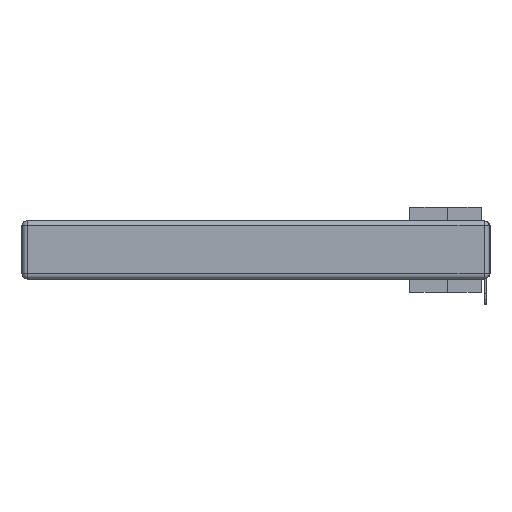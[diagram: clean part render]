
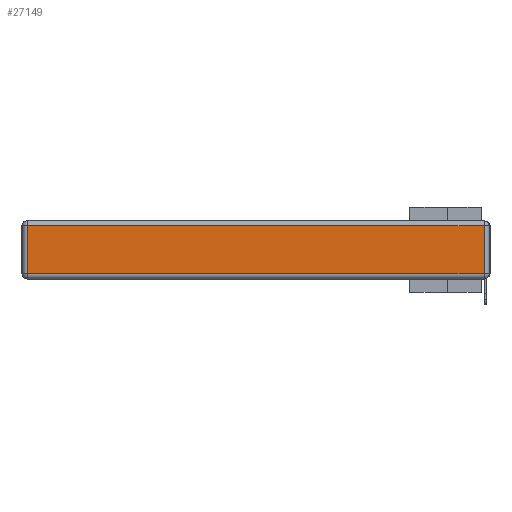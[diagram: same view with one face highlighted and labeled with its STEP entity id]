
A CAD part, left-side view. The second image highlights one B-rep face of the part: STEP entity #27149.
In plain terms, the highlighted planar face has unit normal (-1, 0, 0).
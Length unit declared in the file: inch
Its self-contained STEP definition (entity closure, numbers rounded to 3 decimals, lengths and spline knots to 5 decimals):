
#456 = CARTESIAN_POINT ( 'NONE',  ( 0., 0., -0.313 ) ) ;
#1073 = CARTESIAN_POINT ( 'NONE',  ( 0., 2.72, -0.343 ) ) ;
#1402 = ORIENTED_EDGE ( 'NONE', *, *, #16604, .T. ) ;
#3430 = EDGE_LOOP ( 'NONE', ( #16797, #22699, #1402, #30811 ) ) ;
#3809 = DIRECTION ( 'NONE',  ( 0., 1., 0. ) ) ;
#4510 = VECTOR ( 'NONE', #29214, 39.37008 ) ;
#4762 = CARTESIAN_POINT ( 'NONE',  ( 0., 2.72, -0.03 ) ) ;
#6203 = DIRECTION ( 'NONE',  ( 0., 0., -1. ) ) ;
#6342 = DIRECTION ( 'NONE',  ( 0., 0., 1. ) ) ;
#6616 = VERTEX_POINT ( 'NONE', #13841 ) ;
#13573 = CARTESIAN_POINT ( 'NONE',  ( 0., 0.03, -0.313 ) ) ;
#13841 = CARTESIAN_POINT ( 'NONE',  ( 0., 2.72, -0.313 ) ) ;
#15039 = EDGE_CURVE ( 'NONE', #6616, #26564, #16001, .T. ) ;
#16001 = LINE ( 'NONE', #456, #4510 ) ;
#16604 = EDGE_CURVE ( 'NONE', #32747, #22428, #21941, .T. ) ;
#16797 = ORIENTED_EDGE ( 'NONE', *, *, #15039, .T. ) ;
#17146 = LINE ( 'NONE', #22126, #30282 ) ;
#19828 = PLANE ( 'NONE',  #27016 ) ;
#21829 = EDGE_CURVE ( 'NONE', #22428, #6616, #24355, .T. ) ;
#21941 = LINE ( 'NONE', #32589, #24832 ) ;
#22126 = CARTESIAN_POINT ( 'NONE',  ( 0., 0.03, -0.343 ) ) ;
#22428 = VERTEX_POINT ( 'NONE', #4762 ) ;
#22699 = ORIENTED_EDGE ( 'NONE', *, *, #28020, .T. ) ;
#24355 = LINE ( 'NONE', #1073, #28858 ) ;
#24832 = VECTOR ( 'NONE', #3809, 39.37008 ) ;
#26564 = VERTEX_POINT ( 'NONE', #13573 ) ;
#27016 = AXIS2_PLACEMENT_3D ( 'NONE', #27732, #32885, #6342 ) ;
#27043 = FACE_OUTER_BOUND ( 'NONE', #3430, .T. ) ;
#27149 = ADVANCED_FACE ( 'NONE', ( #27043 ), #19828, .T. ) ;
#27732 = CARTESIAN_POINT ( 'NONE',  ( 0., 0., -0.343 ) ) ;
#28020 = EDGE_CURVE ( 'NONE', #26564, #32747, #17146, .T. ) ;
#28858 = VECTOR ( 'NONE', #6203, 39.37008 ) ;
#29214 = DIRECTION ( 'NONE',  ( 0., -1., 0. ) ) ;
#30106 = CARTESIAN_POINT ( 'NONE',  ( 0., 0.03, -0.03 ) ) ;
#30282 = VECTOR ( 'NONE', #30356, 39.37008 ) ;
#30356 = DIRECTION ( 'NONE',  ( 0., 0., 1. ) ) ;
#30811 = ORIENTED_EDGE ( 'NONE', *, *, #21829, .T. ) ;
#32589 = CARTESIAN_POINT ( 'NONE',  ( 0., 2.75, -0.03 ) ) ;
#32747 = VERTEX_POINT ( 'NONE', #30106 ) ;
#32885 = DIRECTION ( 'NONE',  ( -1., 0., 0. ) ) ;
